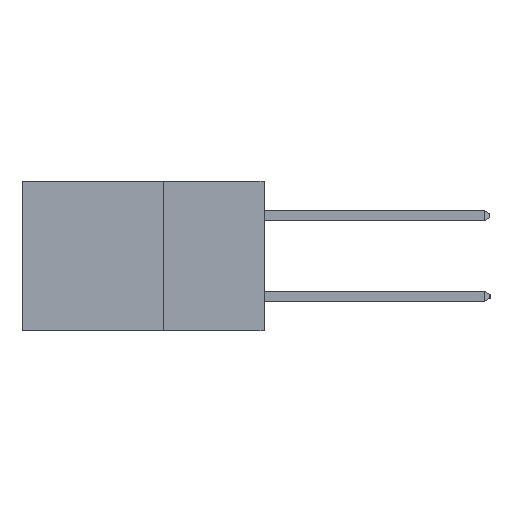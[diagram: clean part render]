
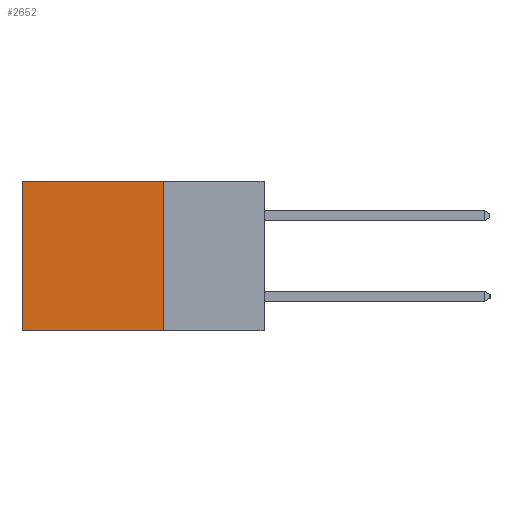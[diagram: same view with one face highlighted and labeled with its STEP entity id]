
A CAD part, left-side view. The second image highlights one B-rep face of the part: STEP entity #2652.
In plain terms, the highlighted planar face has unit normal (-1, 0, 0).
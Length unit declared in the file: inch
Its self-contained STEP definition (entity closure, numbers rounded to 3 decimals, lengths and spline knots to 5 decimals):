
#360 = VERTEX_POINT ( 'NONE', #1371 ) ;
#659 = CARTESIAN_POINT ( 'NONE',  ( 0.2615, 0.6, -0.37 ) ) ;
#866 = CARTESIAN_POINT ( 'NONE',  ( 0.2615, 0.25, 0. ) ) ;
#1365 = VECTOR ( 'NONE', #10489, 39.37008 ) ;
#1371 = CARTESIAN_POINT ( 'NONE',  ( 0.2615, 0.6, -0.37 ) ) ;
#1386 = ORIENTED_EDGE ( 'NONE', *, *, #14525, .T. ) ;
#2240 = ORIENTED_EDGE ( 'NONE', *, *, #8979, .T. ) ;
#2652 = ADVANCED_FACE ( 'NONE', ( #10580 ), #10815, .F. ) ;
#2833 = LINE ( 'NONE', #12980, #15743 ) ;
#3392 = ORIENTED_EDGE ( 'NONE', *, *, #10381, .F. ) ;
#3852 = DIRECTION ( 'NONE',  ( 0., 1., 0. ) ) ;
#4167 = VERTEX_POINT ( 'NONE', #12854 ) ;
#5336 = VECTOR ( 'NONE', #12491, 39.37008 ) ;
#5730 = LINE ( 'NONE', #659, #5336 ) ;
#5755 = VERTEX_POINT ( 'NONE', #866 ) ;
#6529 = EDGE_LOOP ( 'NONE', ( #1386, #3392, #15941, #2240 ) ) ;
#7464 = VERTEX_POINT ( 'NONE', #12184 ) ;
#7976 = CARTESIAN_POINT ( 'NONE',  ( 0.2615, 0.25, -0.37 ) ) ;
#8376 = LINE ( 'NONE', #9177, #1365 ) ;
#8979 = EDGE_CURVE ( 'NONE', #5755, #4167, #2833, .T. ) ;
#9177 = CARTESIAN_POINT ( 'NONE',  ( 0.2615, 0.25, -0.37 ) ) ;
#9366 = VECTOR ( 'NONE', #11940, 39.37008 ) ;
#9712 = EDGE_CURVE ( 'NONE', #5755, #7464, #8376, .T. ) ;
#10381 = EDGE_CURVE ( 'NONE', #7464, #360, #15307, .T. ) ;
#10392 = DIRECTION ( 'NONE',  ( 1., 0., 0. ) ) ;
#10489 = DIRECTION ( 'NONE',  ( 0., 0., -1. ) ) ;
#10580 = FACE_OUTER_BOUND ( 'NONE', #6529, .T. ) ;
#10747 = CARTESIAN_POINT ( 'NONE',  ( 0.2615, 0.25, -0.37 ) ) ;
#10815 = PLANE ( 'NONE',  #14746 ) ;
#11940 = DIRECTION ( 'NONE',  ( 0., 1., 0. ) ) ;
#12184 = CARTESIAN_POINT ( 'NONE',  ( 0.2615, 0.25, -0.37 ) ) ;
#12491 = DIRECTION ( 'NONE',  ( 0., 0., -1. ) ) ;
#12854 = CARTESIAN_POINT ( 'NONE',  ( 0.2615, 0.6, 0. ) ) ;
#12950 = DIRECTION ( 'NONE',  ( 0., 0., -1. ) ) ;
#12980 = CARTESIAN_POINT ( 'NONE',  ( 0.2615, 0.25, 0. ) ) ;
#14525 = EDGE_CURVE ( 'NONE', #4167, #360, #5730, .T. ) ;
#14746 = AXIS2_PLACEMENT_3D ( 'NONE', #10747, #10392, #12950 ) ;
#15307 = LINE ( 'NONE', #7976, #9366 ) ;
#15743 = VECTOR ( 'NONE', #3852, 39.37008 ) ;
#15941 = ORIENTED_EDGE ( 'NONE', *, *, #9712, .F. ) ;
